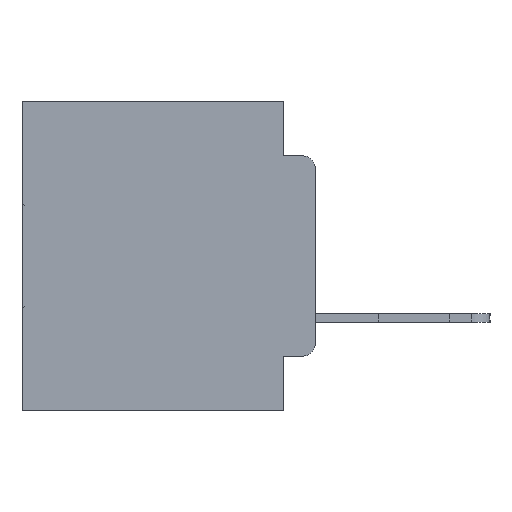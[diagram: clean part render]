
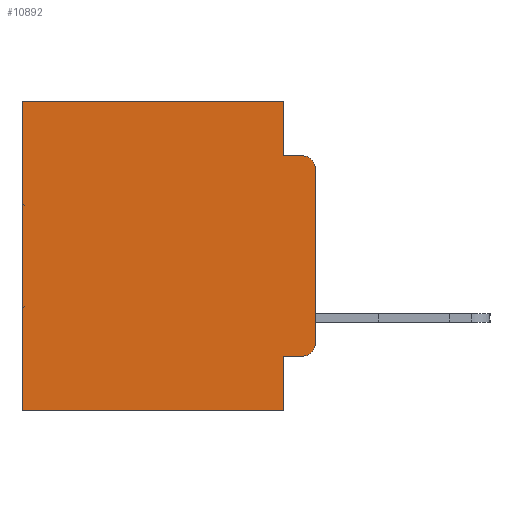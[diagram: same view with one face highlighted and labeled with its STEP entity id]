
A CAD part, left-side view. The second image highlights one B-rep face of the part: STEP entity #10892.
In plain terms, the highlighted planar face has unit normal (-1, 0, 0).
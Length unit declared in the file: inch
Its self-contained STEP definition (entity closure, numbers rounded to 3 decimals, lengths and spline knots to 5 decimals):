
#1206 = ORIENTED_EDGE ( 'NONE', *, *, #24992, .F. ) ;
#1730 = EDGE_CURVE ( 'NONE', #13157, #13992, #18823, .T. ) ;
#1788 = EDGE_CURVE ( 'NONE', #17862, #9041, #23210, .T. ) ;
#2425 = ORIENTED_EDGE ( 'NONE', *, *, #15205, .T. ) ;
#2933 = VECTOR ( 'NONE', #29611, 39.37008 ) ;
#3078 = LINE ( 'NONE', #6401, #15832 ) ;
#3132 = CARTESIAN_POINT ( 'NONE',  ( 0.298, 0.02, -0.1085 ) ) ;
#3737 = CARTESIAN_POINT ( 'NONE',  ( 0.298, 0.473, 0. ) ) ;
#3999 = DIRECTION ( 'NONE',  ( 0., 0., -1. ) ) ;
#4084 = AXIS2_PLACEMENT_3D ( 'NONE', #9981, #21274, #3999 ) ;
#4238 = DIRECTION ( 'NONE',  ( -1., 0., 0. ) ) ;
#4272 = VECTOR ( 'NONE', #7416, 39.37008 ) ;
#4307 = CARTESIAN_POINT ( 'NONE',  ( 0.298, 0., -0.1085 ) ) ;
#5129 = EDGE_CURVE ( 'NONE', #27403, #13157, #30960, .T. ) ;
#5160 = VERTEX_POINT ( 'NONE', #3737 ) ;
#5217 = ORIENTED_EDGE ( 'NONE', *, *, #17149, .T. ) ;
#5493 = VERTEX_POINT ( 'NONE', #5597 ) ;
#5597 = CARTESIAN_POINT ( 'NONE',  ( 0.298, 0., -0.3915 ) ) ;
#5642 = DIRECTION ( 'NONE',  ( 0., 0., -1. ) ) ;
#5949 = CARTESIAN_POINT ( 'NONE',  ( 0.298, 0.051, -0.5 ) ) ;
#6371 = LINE ( 'NONE', #19028, #25057 ) ;
#6401 = CARTESIAN_POINT ( 'NONE',  ( 0.298, 0.473, 0. ) ) ;
#6760 = EDGE_CURVE ( 'NONE', #27403, #5160, #19295, .T. ) ;
#7416 = DIRECTION ( 'NONE',  ( 0., 0., -1. ) ) ;
#7944 = ORIENTED_EDGE ( 'NONE', *, *, #6760, .T. ) ;
#8951 = DIRECTION ( 'NONE',  ( 0., 0., -1. ) ) ;
#9041 = VERTEX_POINT ( 'NONE', #5949 ) ;
#9696 = CARTESIAN_POINT ( 'NONE',  ( 0.298, 0.051, -0.0885 ) ) ;
#9842 = VECTOR ( 'NONE', #28404, 39.37008 ) ;
#9981 = CARTESIAN_POINT ( 'NONE',  ( 0.298, 0., 0. ) ) ;
#10444 = EDGE_CURVE ( 'NONE', #17862, #12016, #20297, .T. ) ;
#10493 = VERTEX_POINT ( 'NONE', #17724 ) ;
#10766 = EDGE_CURVE ( 'NONE', #29235, #5493, #16750, .T. ) ;
#10892 = ADVANCED_FACE ( 'NONE', ( #12679 ), #19344, .F. ) ;
#12016 = VERTEX_POINT ( 'NONE', #14611 ) ;
#12192 = DIRECTION ( 'NONE',  ( 0., 1., 0. ) ) ;
#12495 = VECTOR ( 'NONE', #12192, 39.37008 ) ;
#12679 = FACE_OUTER_BOUND ( 'NONE', #19404, .T. ) ;
#12847 = CIRCLE ( 'NONE', #28935, 0.02 ) ;
#13157 = VERTEX_POINT ( 'NONE', #9696 ) ;
#13506 = CARTESIAN_POINT ( 'NONE',  ( 0.298, 0.02, -0.0885 ) ) ;
#13992 = VERTEX_POINT ( 'NONE', #13506 ) ;
#14611 = CARTESIAN_POINT ( 'NONE',  ( 0.298, 0.02, -0.4115 ) ) ;
#14705 = CARTESIAN_POINT ( 'NONE',  ( 0.298, 0.051, 0. ) ) ;
#15205 = EDGE_CURVE ( 'NONE', #5160, #10493, #3078, .T. ) ;
#15738 = DIRECTION ( 'NONE',  ( 0., -1., 0. ) ) ;
#15831 = CARTESIAN_POINT ( 'NONE',  ( 0.298, 0., 0. ) ) ;
#15832 = VECTOR ( 'NONE', #8951, 39.37008 ) ;
#16463 = VECTOR ( 'NONE', #21587, 39.37008 ) ;
#16750 = LINE ( 'NONE', #15831, #9842 ) ;
#17149 = EDGE_CURVE ( 'NONE', #12016, #5493, #12847, .T. ) ;
#17724 = CARTESIAN_POINT ( 'NONE',  ( 0.298, 0.473, -0.5 ) ) ;
#17862 = VERTEX_POINT ( 'NONE', #20817 ) ;
#18823 = LINE ( 'NONE', #27127, #26269 ) ;
#19028 = CARTESIAN_POINT ( 'NONE',  ( 0.298, 0., -0.5 ) ) ;
#19295 = LINE ( 'NONE', #20745, #12495 ) ;
#19344 = PLANE ( 'NONE',  #4084 ) ;
#19404 = EDGE_LOOP ( 'NONE', ( #21092, #26533, #30737, #21509, #7944, #2425, #1206, #32222, #31092, #5217 ) ) ;
#19411 = EDGE_CURVE ( 'NONE', #29235, #13992, #30366, .T. ) ;
#19460 = CARTESIAN_POINT ( 'NONE',  ( 0.298, 0.02, -0.3915 ) ) ;
#20297 = LINE ( 'NONE', #31318, #16463 ) ;
#20745 = CARTESIAN_POINT ( 'NONE',  ( 0.298, 0., 0. ) ) ;
#20817 = CARTESIAN_POINT ( 'NONE',  ( 0.298, 0.051, -0.4115 ) ) ;
#20893 = DIRECTION ( 'NONE',  ( -1., 0., 0. ) ) ;
#21092 = ORIENTED_EDGE ( 'NONE', *, *, #10766, .F. ) ;
#21274 = DIRECTION ( 'NONE',  ( 1., 0., 0. ) ) ;
#21509 = ORIENTED_EDGE ( 'NONE', *, *, #5129, .F. ) ;
#21576 = DIRECTION ( 'NONE',  ( 0., 1., 0. ) ) ;
#21587 = DIRECTION ( 'NONE',  ( 0., -1., 0. ) ) ;
#21990 = DIRECTION ( 'NONE',  ( 0., 0., -1. ) ) ;
#22414 = AXIS2_PLACEMENT_3D ( 'NONE', #3132, #20893, #5642 ) ;
#23210 = LINE ( 'NONE', #27091, #2933 ) ;
#24992 = EDGE_CURVE ( 'NONE', #9041, #10493, #6371, .T. ) ;
#25057 = VECTOR ( 'NONE', #21576, 39.37008 ) ;
#26269 = VECTOR ( 'NONE', #15738, 39.37008 ) ;
#26533 = ORIENTED_EDGE ( 'NONE', *, *, #19411, .T. ) ;
#27091 = CARTESIAN_POINT ( 'NONE',  ( 0.298, 0.051, 0. ) ) ;
#27127 = CARTESIAN_POINT ( 'NONE',  ( 0.298, 0.051, -0.0885 ) ) ;
#27132 = CARTESIAN_POINT ( 'NONE',  ( 0.298, 0.051, 0. ) ) ;
#27403 = VERTEX_POINT ( 'NONE', #14705 ) ;
#28404 = DIRECTION ( 'NONE',  ( 0., 0., -1. ) ) ;
#28935 = AXIS2_PLACEMENT_3D ( 'NONE', #19460, #4238, #21990 ) ;
#29235 = VERTEX_POINT ( 'NONE', #4307 ) ;
#29611 = DIRECTION ( 'NONE',  ( 0., 0., -1. ) ) ;
#30366 = CIRCLE ( 'NONE', #22414, 0.02 ) ;
#30737 = ORIENTED_EDGE ( 'NONE', *, *, #1730, .F. ) ;
#30960 = LINE ( 'NONE', #27132, #4272 ) ;
#31092 = ORIENTED_EDGE ( 'NONE', *, *, #10444, .T. ) ;
#31318 = CARTESIAN_POINT ( 'NONE',  ( 0.298, 0.051, -0.4115 ) ) ;
#32222 = ORIENTED_EDGE ( 'NONE', *, *, #1788, .F. ) ;
